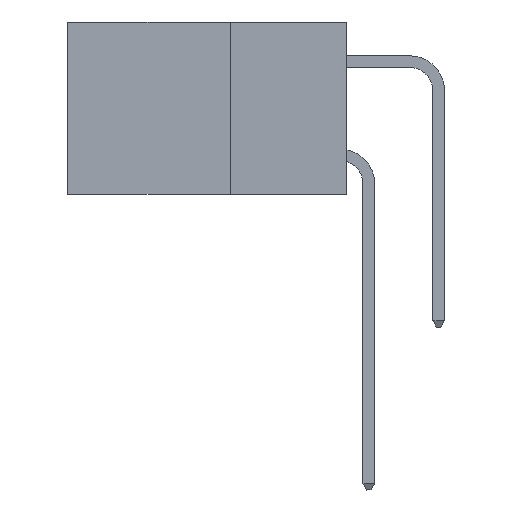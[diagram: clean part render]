
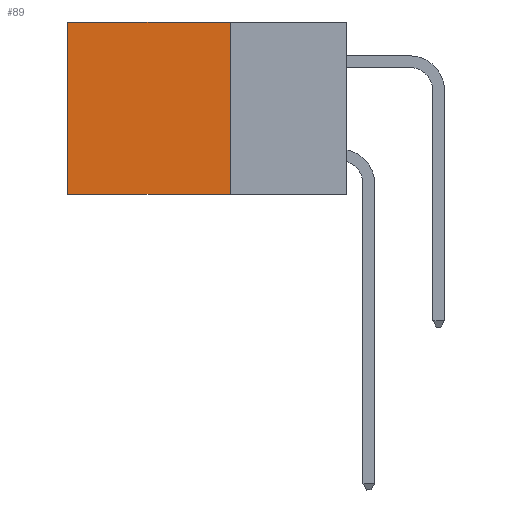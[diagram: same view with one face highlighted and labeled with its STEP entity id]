
A CAD part, left-side view. The second image highlights one B-rep face of the part: STEP entity #89.
In plain terms, the highlighted planar face has unit normal (-1, 0, 0).
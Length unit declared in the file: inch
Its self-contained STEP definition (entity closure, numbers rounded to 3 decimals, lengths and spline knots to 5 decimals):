
#89 = ADVANCED_FACE ( 'NONE', ( #15501 ), #6888, .F. ) ;
#415 = AXIS2_PLACEMENT_3D ( 'NONE', #6854, #10138, #8680 ) ;
#2069 = LINE ( 'NONE', #7373, #23960 ) ;
#2143 = CARTESIAN_POINT ( 'NONE',  ( 0.2875, 0.25, -0.37 ) ) ;
#2190 = CARTESIAN_POINT ( 'NONE',  ( 0.2875, 0.25, 0. ) ) ;
#2703 = VERTEX_POINT ( 'NONE', #10528 ) ;
#5293 = DIRECTION ( 'NONE',  ( 0., 0., -1. ) ) ;
#5341 = DIRECTION ( 'NONE',  ( 0., 1., 0. ) ) ;
#5549 = VECTOR ( 'NONE', #21763, 39.37008 ) ;
#6854 = CARTESIAN_POINT ( 'NONE',  ( 0.2875, 0.25, 0. ) ) ;
#6888 = PLANE ( 'NONE',  #415 ) ;
#7373 = CARTESIAN_POINT ( 'NONE',  ( 0.2875, 0.25, -0.37 ) ) ;
#8680 = DIRECTION ( 'NONE',  ( 0., 0., -1. ) ) ;
#8789 = LINE ( 'NONE', #2190, #20091 ) ;
#8909 = VECTOR ( 'NONE', #5293, 39.37008 ) ;
#10138 = DIRECTION ( 'NONE',  ( 1., 0., 0. ) ) ;
#10528 = CARTESIAN_POINT ( 'NONE',  ( 0.2875, 0.25, 0. ) ) ;
#11174 = LINE ( 'NONE', #23703, #5549 ) ;
#11625 = EDGE_CURVE ( 'NONE', #16900, #14179, #25745, .T. ) ;
#13422 = EDGE_CURVE ( 'NONE', #2703, #16900, #11174, .T. ) ;
#14179 = VERTEX_POINT ( 'NONE', #24870 ) ;
#15282 = EDGE_CURVE ( 'NONE', #16997, #14179, #2069, .T. ) ;
#15501 = FACE_OUTER_BOUND ( 'NONE', #26608, .T. ) ;
#16900 = VERTEX_POINT ( 'NONE', #18907 ) ;
#16997 = VERTEX_POINT ( 'NONE', #2143 ) ;
#17110 = DIRECTION ( 'NONE',  ( 0., 0., -1. ) ) ;
#18040 = CARTESIAN_POINT ( 'NONE',  ( 0.2875, 0.6, 0. ) ) ;
#18907 = CARTESIAN_POINT ( 'NONE',  ( 0.2875, 0.6, 0. ) ) ;
#20091 = VECTOR ( 'NONE', #17110, 39.37008 ) ;
#21630 = ORIENTED_EDGE ( 'NONE', *, *, #15282, .F. ) ;
#21763 = DIRECTION ( 'NONE',  ( 0., 1., 0. ) ) ;
#21867 = ORIENTED_EDGE ( 'NONE', *, *, #13422, .T. ) ;
#22386 = ORIENTED_EDGE ( 'NONE', *, *, #11625, .T. ) ;
#23703 = CARTESIAN_POINT ( 'NONE',  ( 0.2875, 0.25, 0. ) ) ;
#23960 = VECTOR ( 'NONE', #5341, 39.37008 ) ;
#24222 = ORIENTED_EDGE ( 'NONE', *, *, #26259, .F. ) ;
#24870 = CARTESIAN_POINT ( 'NONE',  ( 0.2875, 0.6, -0.37 ) ) ;
#25745 = LINE ( 'NONE', #18040, #8909 ) ;
#26259 = EDGE_CURVE ( 'NONE', #2703, #16997, #8789, .T. ) ;
#26608 = EDGE_LOOP ( 'NONE', ( #22386, #21630, #24222, #21867 ) ) ;
